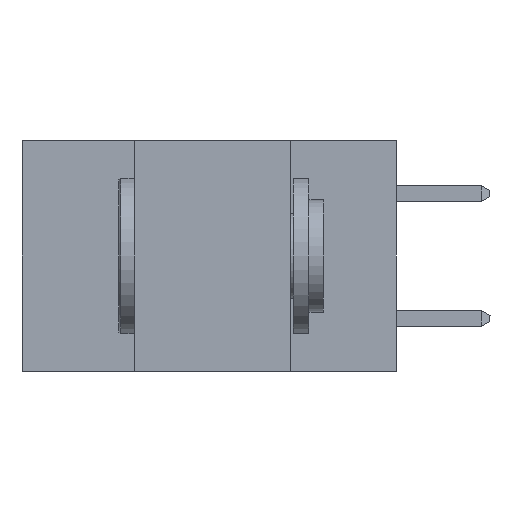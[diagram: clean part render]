
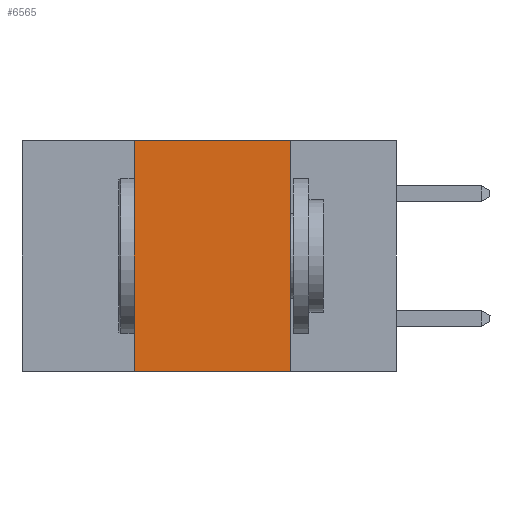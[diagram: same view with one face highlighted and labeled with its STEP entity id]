
A CAD part, left-side view. The second image highlights one B-rep face of the part: STEP entity #6565.
In plain terms, the highlighted planar face has unit normal (-1, 0, 0).
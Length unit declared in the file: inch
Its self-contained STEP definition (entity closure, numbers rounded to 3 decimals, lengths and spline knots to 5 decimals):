
#184 = EDGE_CURVE ( 'NONE', #1748, #7365, #229, .T. ) ;
#229 = LINE ( 'NONE', #4724, #8928 ) ;
#1329 = VECTOR ( 'NONE', #6722, 39.37008 ) ;
#1748 = VERTEX_POINT ( 'NONE', #10927 ) ;
#1763 = EDGE_CURVE ( 'NONE', #2363, #7907, #9036, .T. ) ;
#2223 = EDGE_CURVE ( 'NONE', #7907, #1748, #6342, .T. ) ;
#2363 = VERTEX_POINT ( 'NONE', #3380 ) ;
#2620 = ORIENTED_EDGE ( 'NONE', *, *, #184, .F. ) ;
#3380 = CARTESIAN_POINT ( 'NONE',  ( 0., 0.42, -0.37 ) ) ;
#4406 = ORIENTED_EDGE ( 'NONE', *, *, #4625, .T. ) ;
#4625 = EDGE_CURVE ( 'NONE', #2363, #7365, #11274, .T. ) ;
#4658 = PLANE ( 'NONE',  #7431 ) ;
#4671 = DIRECTION ( 'NONE',  ( 0., 0., -1. ) ) ;
#4701 = DIRECTION ( 'NONE',  ( 1., 0., 0. ) ) ;
#4724 = CARTESIAN_POINT ( 'NONE',  ( 0., 0.17, -0.37 ) ) ;
#4727 = DIRECTION ( 'NONE',  ( 0., 0., -1. ) ) ;
#4830 = ORIENTED_EDGE ( 'NONE', *, *, #1763, .F. ) ;
#5024 = CARTESIAN_POINT ( 'NONE',  ( 0., 0.6, 0. ) ) ;
#6342 = LINE ( 'NONE', #6648, #11419 ) ;
#6565 = ADVANCED_FACE ( 'NONE', ( #10492 ), #4658, .F. ) ;
#6648 = CARTESIAN_POINT ( 'NONE',  ( 0., 0.6, 0. ) ) ;
#6722 = DIRECTION ( 'NONE',  ( 0., 0., 1. ) ) ;
#6732 = DIRECTION ( 'NONE',  ( 0., -1., 0. ) ) ;
#7365 = VERTEX_POINT ( 'NONE', #10417 ) ;
#7399 = CARTESIAN_POINT ( 'NONE',  ( 0., 0.42, 0. ) ) ;
#7431 = AXIS2_PLACEMENT_3D ( 'NONE', #5024, #4701, #4727 ) ;
#7749 = CARTESIAN_POINT ( 'NONE',  ( 0., 0.42, -0.37 ) ) ;
#7907 = VERTEX_POINT ( 'NONE', #7399 ) ;
#8151 = CARTESIAN_POINT ( 'NONE',  ( 0., 0.6, -0.37 ) ) ;
#8303 = DIRECTION ( 'NONE',  ( 0., -1., 0. ) ) ;
#8928 = VECTOR ( 'NONE', #4671, 39.37008 ) ;
#8931 = ORIENTED_EDGE ( 'NONE', *, *, #2223, .F. ) ;
#9036 = LINE ( 'NONE', #7749, #1329 ) ;
#10133 = EDGE_LOOP ( 'NONE', ( #2620, #8931, #4830, #4406 ) ) ;
#10417 = CARTESIAN_POINT ( 'NONE',  ( 0., 0.17, -0.37 ) ) ;
#10492 = FACE_OUTER_BOUND ( 'NONE', #10133, .T. ) ;
#10927 = CARTESIAN_POINT ( 'NONE',  ( 0., 0.17, 0. ) ) ;
#10977 = VECTOR ( 'NONE', #8303, 39.37008 ) ;
#11274 = LINE ( 'NONE', #8151, #10977 ) ;
#11419 = VECTOR ( 'NONE', #6732, 39.37008 ) ;
